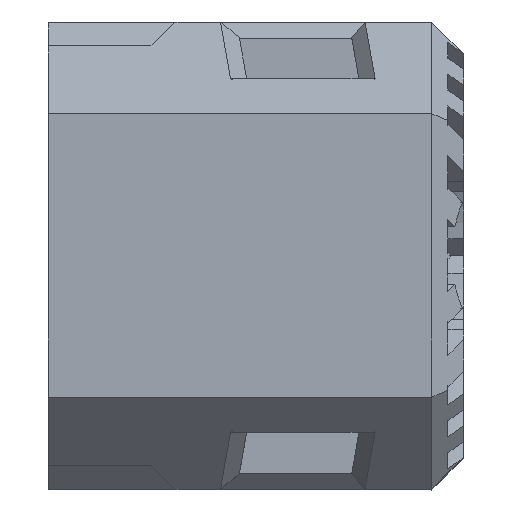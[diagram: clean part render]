
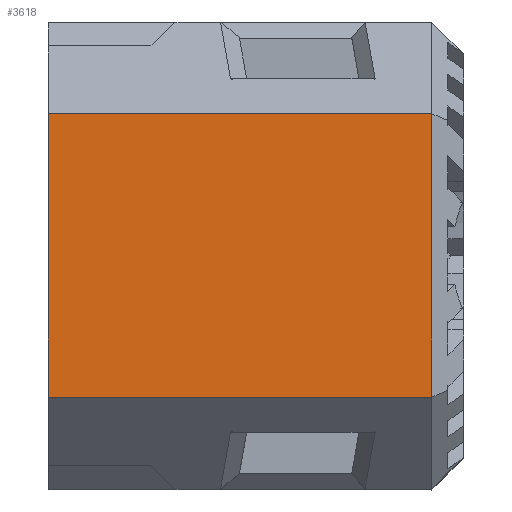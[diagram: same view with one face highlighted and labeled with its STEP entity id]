
A CAD part, top view. The second image highlights one B-rep face of the part: STEP entity #3618.
In plain terms, the highlighted planar face has unit normal (0, 0, 1).
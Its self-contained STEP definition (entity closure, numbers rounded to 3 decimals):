
#125=LINE('',#5149,#558);
#214=LINE('',#5342,#647);
#227=LINE('',#5374,#660);
#447=LINE('',#5895,#880);
#558=VECTOR('',#4144,10.);
#647=VECTOR('',#4307,10.);
#660=VECTOR('',#4340,10.);
#880=VECTOR('',#4842,10.);
#1107=FACE_OUTER_BOUND('',#1302,.T.);
#1302=EDGE_LOOP('',(#3264,#3265,#3266,#3267));
#1474=VERTEX_POINT('',#5146);
#1475=VERTEX_POINT('',#5148);
#1542=VERTEX_POINT('',#5341);
#1551=VERTEX_POINT('',#5372);
#1844=EDGE_CURVE('',#1474,#1475,#125,.T.);
#1940=EDGE_CURVE('',#1542,#1475,#214,.T.);
#1958=EDGE_CURVE('',#1551,#1474,#227,.T.);
#2220=EDGE_CURVE('',#1542,#1551,#447,.T.);
#3264=ORIENTED_EDGE('',*,*,#2220,.F.);
#3265=ORIENTED_EDGE('',*,*,#1940,.T.);
#3266=ORIENTED_EDGE('',*,*,#1844,.F.);
#3267=ORIENTED_EDGE('',*,*,#1958,.F.);
#3431=PLANE('',#3905);
#3618=ADVANCED_FACE('',(#1107),#3431,.T.);
#3905=AXIS2_PLACEMENT_3D('',#5925,#4884,#4885);
#4144=DIRECTION('',(0.,1.,0.));
#4307=DIRECTION('',(-1.,0.,0.));
#4340=DIRECTION('',(-1.,0.,0.));
#4842=DIRECTION('',(0.,-1.,0.));
#4884=DIRECTION('center_axis',(0.,0.,
1.));
#4885=DIRECTION('ref_axis',(0.,-1.,0.));
#5146=CARTESIAN_POINT('',(180.135,-132.355,-1.747));
#5148=CARTESIAN_POINT('',(180.135,-114.623,-1.747));
#5149=CARTESIAN_POINT('',(180.135,-115.876,-1.747));
#5341=CARTESIAN_POINT('',(204.135,-114.623,-1.747));
#5342=CARTESIAN_POINT('',(185.135,-114.623,-1.747));
#5372=CARTESIAN_POINT('',(204.135,-132.355,-1.747));
#5374=CARTESIAN_POINT('',(48.255,-132.355,-1.747));
#5895=CARTESIAN_POINT('',(204.135,-122.434,-1.747));
#5925=CARTESIAN_POINT('Origin',(-22.625,-108.264,-1.747));
